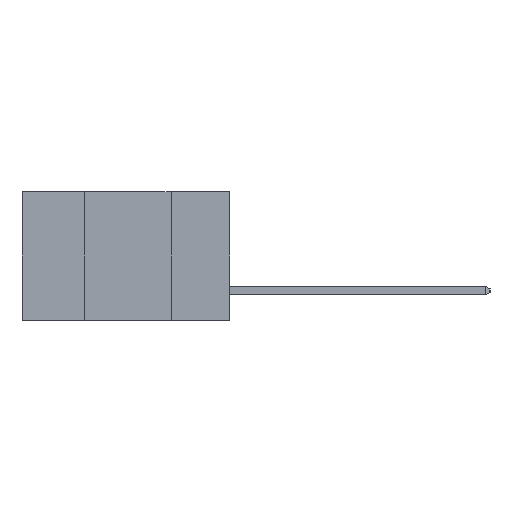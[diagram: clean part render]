
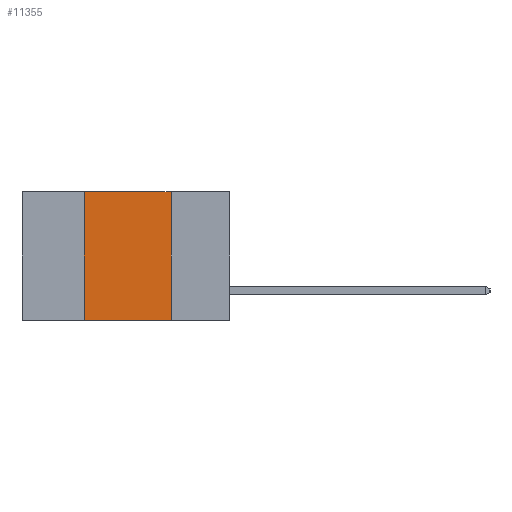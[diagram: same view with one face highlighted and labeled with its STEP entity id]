
A CAD part, left-side view. The second image highlights one B-rep face of the part: STEP entity #11355.
In plain terms, the highlighted planar face has unit normal (-1, 0, 0).
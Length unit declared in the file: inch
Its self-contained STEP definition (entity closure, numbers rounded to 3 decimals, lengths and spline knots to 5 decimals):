
#1435 = VECTOR ( 'NONE', #13205, 39.37008 ) ;
#1620 = VERTEX_POINT ( 'NONE', #5351 ) ;
#1860 = FACE_OUTER_BOUND ( 'NONE', #24777, .T. ) ;
#2740 = EDGE_CURVE ( 'NONE', #5179, #1620, #23934, .T. ) ;
#2916 = CARTESIAN_POINT ( 'NONE',  ( 0., 0.6, 0. ) ) ;
#3165 = EDGE_CURVE ( 'NONE', #23985, #5079, #12598, .T. ) ;
#4992 = DIRECTION ( 'NONE',  ( 0., 0., 1. ) ) ;
#5079 = VERTEX_POINT ( 'NONE', #15570 ) ;
#5179 = VERTEX_POINT ( 'NONE', #25547 ) ;
#5351 = CARTESIAN_POINT ( 'NONE',  ( 0., 0.42, 0. ) ) ;
#5411 = DIRECTION ( 'NONE',  ( 0., 0., -1. ) ) ;
#10731 = CARTESIAN_POINT ( 'NONE',  ( 0., 0.6, -0.37 ) ) ;
#11355 = ADVANCED_FACE ( 'NONE', ( #1860 ), #24698, .F. ) ;
#11386 = DIRECTION ( 'NONE',  ( 0., 0., -1. ) ) ;
#11883 = CARTESIAN_POINT ( 'NONE',  ( 0., 0.17, 0. ) ) ;
#12598 = LINE ( 'NONE', #11883, #23909 ) ;
#12847 = CARTESIAN_POINT ( 'NONE',  ( 0., 0.6, 0. ) ) ;
#13205 = DIRECTION ( 'NONE',  ( 0., -1., 0. ) ) ;
#13232 = CARTESIAN_POINT ( 'NONE',  ( 0., 0.17, 0. ) ) ;
#13341 = AXIS2_PLACEMENT_3D ( 'NONE', #2916, #19983, #5411 ) ;
#14475 = LINE ( 'NONE', #10731, #1435 ) ;
#15238 = ORIENTED_EDGE ( 'NONE', *, *, #3165, .F. ) ;
#15570 = CARTESIAN_POINT ( 'NONE',  ( 0., 0.17, -0.37 ) ) ;
#16044 = EDGE_CURVE ( 'NONE', #5179, #5079, #14475, .T. ) ;
#16685 = EDGE_CURVE ( 'NONE', #1620, #23985, #21211, .T. ) ;
#19340 = ORIENTED_EDGE ( 'NONE', *, *, #2740, .F. ) ;
#19983 = DIRECTION ( 'NONE',  ( 1., 0., 0. ) ) ;
#21211 = LINE ( 'NONE', #12847, #26815 ) ;
#23720 = CARTESIAN_POINT ( 'NONE',  ( 0., 0.42, 0. ) ) ;
#23909 = VECTOR ( 'NONE', #11386, 39.37008 ) ;
#23934 = LINE ( 'NONE', #23720, #29510 ) ;
#23985 = VERTEX_POINT ( 'NONE', #13232 ) ;
#24332 = ORIENTED_EDGE ( 'NONE', *, *, #16044, .T. ) ;
#24698 = PLANE ( 'NONE',  #13341 ) ;
#24777 = EDGE_LOOP ( 'NONE', ( #15238, #27499, #19340, #24332 ) ) ;
#24812 = DIRECTION ( 'NONE',  ( 0., -1., 0. ) ) ;
#25547 = CARTESIAN_POINT ( 'NONE',  ( 0., 0.42, -0.37 ) ) ;
#26815 = VECTOR ( 'NONE', #24812, 39.37008 ) ;
#27499 = ORIENTED_EDGE ( 'NONE', *, *, #16685, .F. ) ;
#29510 = VECTOR ( 'NONE', #4992, 39.37008 ) ;
